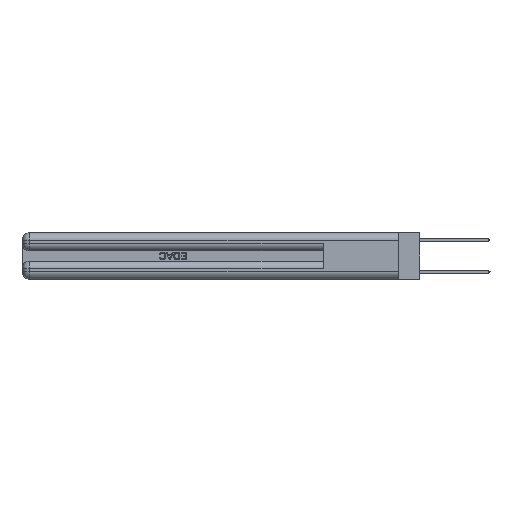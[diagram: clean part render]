
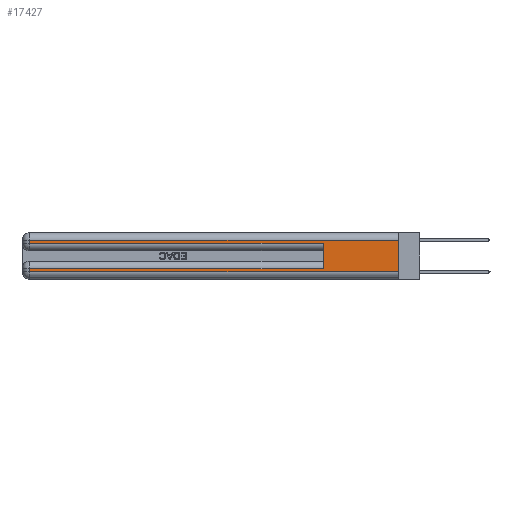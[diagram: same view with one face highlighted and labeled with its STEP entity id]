
A CAD part, left-side view. The second image highlights one B-rep face of the part: STEP entity #17427.
In plain terms, the highlighted planar face has unit normal (-1, 0, 0).
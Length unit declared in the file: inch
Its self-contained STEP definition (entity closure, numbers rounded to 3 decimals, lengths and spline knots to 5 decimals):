
#274 = VECTOR ( 'NONE', #26146, 39.37008 ) ;
#319 = CARTESIAN_POINT ( 'NONE',  ( 0., 2.94, 0.37 ) ) ;
#503 = CARTESIAN_POINT ( 'NONE',  ( 0., 0.6, 0.285 ) ) ;
#883 = VERTEX_POINT ( 'NONE', #15924 ) ;
#1153 = DIRECTION ( 'NONE',  ( 0., 0., 1. ) ) ;
#1434 = VERTEX_POINT ( 'NONE', #2612 ) ;
#1540 = VECTOR ( 'NONE', #21148, 39.37008 ) ;
#1793 = DIRECTION ( 'NONE',  ( 0., 0., -1. ) ) ;
#2612 = CARTESIAN_POINT ( 'NONE',  ( 0., 0., 0.06 ) ) ;
#4036 = DIRECTION ( 'NONE',  ( 0., 0., -1. ) ) ;
#5246 = VECTOR ( 'NONE', #7144, 39.37008 ) ;
#5788 = VERTEX_POINT ( 'NONE', #503 ) ;
#6815 = CARTESIAN_POINT ( 'NONE',  ( 0., 0., 0.37 ) ) ;
#6915 = EDGE_CURVE ( 'NONE', #29615, #1434, #18519, .T. ) ;
#7144 = DIRECTION ( 'NONE',  ( 0., -1., 0. ) ) ;
#7373 = CARTESIAN_POINT ( 'NONE',  ( 0., 2.94, 0.085 ) ) ;
#7612 = CARTESIAN_POINT ( 'NONE',  ( 0., 0., 0.31 ) ) ;
#9498 = LINE ( 'NONE', #34299, #1540 ) ;
#10291 = CARTESIAN_POINT ( 'NONE',  ( 0., 0., 0.085 ) ) ;
#10660 = VECTOR ( 'NONE', #14599, 39.37008 ) ;
#10939 = DIRECTION ( 'NONE',  ( 0., 0., -1. ) ) ;
#11763 = ORIENTED_EDGE ( 'NONE', *, *, #6915, .T. ) ;
#12111 = VERTEX_POINT ( 'NONE', #32227 ) ;
#12421 = PLANE ( 'NONE',  #13654 ) ;
#12551 = VERTEX_POINT ( 'NONE', #7373 ) ;
#13654 = AXIS2_PLACEMENT_3D ( 'NONE', #22929, #17739, #1793 ) ;
#13915 = EDGE_CURVE ( 'NONE', #883, #12551, #14463, .T. ) ;
#13937 = ORIENTED_EDGE ( 'NONE', *, *, #33227, .F. ) ;
#14463 = LINE ( 'NONE', #10291, #274 ) ;
#14599 = DIRECTION ( 'NONE',  ( 0., 0., -1. ) ) ;
#14620 = EDGE_CURVE ( 'NONE', #12551, #29615, #21031, .T. ) ;
#14831 = VECTOR ( 'NONE', #10939, 39.37008 ) ;
#15663 = VECTOR ( 'NONE', #23468, 39.37008 ) ;
#15924 = CARTESIAN_POINT ( 'NONE',  ( 0., 0.6, 0.085 ) ) ;
#16227 = ORIENTED_EDGE ( 'NONE', *, *, #22406, .F. ) ;
#16930 = CARTESIAN_POINT ( 'NONE',  ( 0., 0., 0.31 ) ) ;
#17104 = CARTESIAN_POINT ( 'NONE',  ( 0., 0.6, 0.145 ) ) ;
#17427 = ADVANCED_FACE ( 'NONE', ( #29507 ), #12421, .F. ) ;
#17739 = DIRECTION ( 'NONE',  ( 1., 0., 0. ) ) ;
#18519 = LINE ( 'NONE', #22999, #5246 ) ;
#18944 = ORIENTED_EDGE ( 'NONE', *, *, #14620, .T. ) ;
#19433 = EDGE_CURVE ( 'NONE', #12111, #25677, #23922, .T. ) ;
#19908 = CARTESIAN_POINT ( 'NONE',  ( 0., 2.94, 0.37 ) ) ;
#20501 = ORIENTED_EDGE ( 'NONE', *, *, #19433, .T. ) ;
#21031 = LINE ( 'NONE', #319, #14831 ) ;
#21148 = DIRECTION ( 'NONE',  ( 0., -1., 0. ) ) ;
#22406 = EDGE_CURVE ( 'NONE', #24571, #1434, #28320, .T. ) ;
#22685 = LINE ( 'NONE', #7612, #15663 ) ;
#22929 = CARTESIAN_POINT ( 'NONE',  ( 0., 0., 0.37 ) ) ;
#22999 = CARTESIAN_POINT ( 'NONE',  ( 0., 0., 0.06 ) ) ;
#23468 = DIRECTION ( 'NONE',  ( 0., 1., 0. ) ) ;
#23922 = LINE ( 'NONE', #19908, #10660 ) ;
#24571 = VERTEX_POINT ( 'NONE', #16930 ) ;
#25677 = VERTEX_POINT ( 'NONE', #32674 ) ;
#26146 = DIRECTION ( 'NONE',  ( 0., 1., 0. ) ) ;
#26272 = ORIENTED_EDGE ( 'NONE', *, *, #13915, .T. ) ;
#27086 = LINE ( 'NONE', #17104, #34092 ) ;
#27228 = EDGE_CURVE ( 'NONE', #25677, #5788, #9498, .T. ) ;
#27483 = VECTOR ( 'NONE', #4036, 39.37008 ) ;
#28320 = LINE ( 'NONE', #6815, #27483 ) ;
#28862 = CARTESIAN_POINT ( 'NONE',  ( 0., 2.94, 0.06 ) ) ;
#28898 = EDGE_CURVE ( 'NONE', #24571, #12111, #22685, .T. ) ;
#29507 = FACE_OUTER_BOUND ( 'NONE', #29817, .T. ) ;
#29615 = VERTEX_POINT ( 'NONE', #28862 ) ;
#29817 = EDGE_LOOP ( 'NONE', ( #16227, #31507, #20501, #31071, #13937, #26272, #18944, #11763 ) ) ;
#31071 = ORIENTED_EDGE ( 'NONE', *, *, #27228, .T. ) ;
#31507 = ORIENTED_EDGE ( 'NONE', *, *, #28898, .T. ) ;
#32227 = CARTESIAN_POINT ( 'NONE',  ( 0., 2.94, 0.31 ) ) ;
#32674 = CARTESIAN_POINT ( 'NONE',  ( 0., 2.94, 0.285 ) ) ;
#33227 = EDGE_CURVE ( 'NONE', #883, #5788, #27086, .T. ) ;
#34092 = VECTOR ( 'NONE', #1153, 39.37008 ) ;
#34299 = CARTESIAN_POINT ( 'NONE',  ( 0., 0., 0.285 ) ) ;
